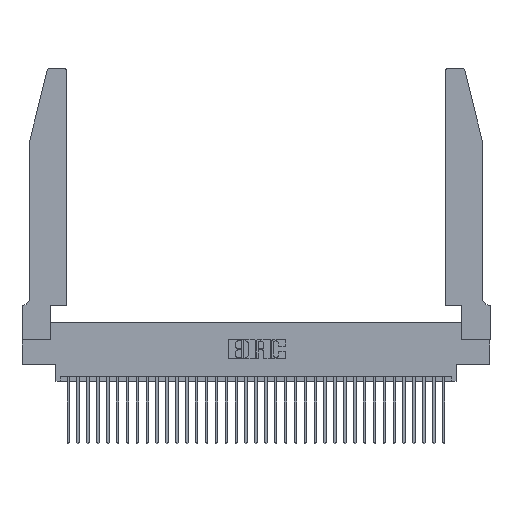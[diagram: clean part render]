
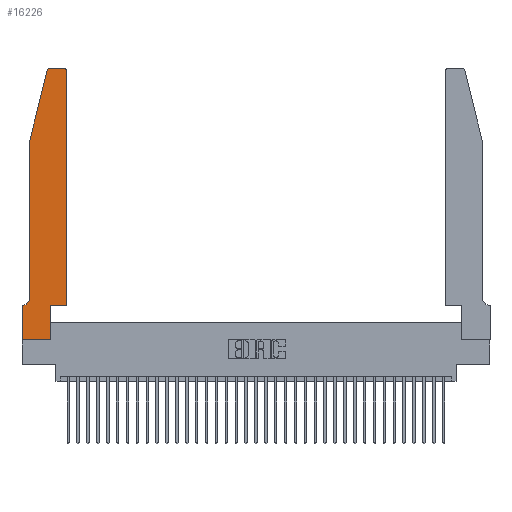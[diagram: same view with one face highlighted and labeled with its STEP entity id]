
A CAD part, top view. The second image highlights one B-rep face of the part: STEP entity #16226.
In plain terms, the highlighted planar face has unit normal (0, 0, 1).
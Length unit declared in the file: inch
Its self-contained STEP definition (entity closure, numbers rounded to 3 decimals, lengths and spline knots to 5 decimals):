
#442 = VERTEX_POINT ( 'NONE', #21804 ) ;
#1699 = ORIENTED_EDGE ( 'NONE', *, *, #30602, .T. ) ;
#1882 = AXIS2_PLACEMENT_3D ( 'NONE', #15471, #9802, #29701 ) ;
#3383 = EDGE_CURVE ( 'NONE', #442, #19058, #23968, .T. ) ;
#3510 = ORIENTED_EDGE ( 'NONE', *, *, #5748, .T. ) ;
#3733 = CARTESIAN_POINT ( 'NONE',  ( 0.4505, 0.35, 0.37 ) ) ;
#4186 = ORIENTED_EDGE ( 'NONE', *, *, #34453, .T. ) ;
#4573 = EDGE_CURVE ( 'NONE', #18616, #24923, #19539, .T. ) ;
#4771 = DIRECTION ( 'NONE',  ( -1., 0., 0. ) ) ;
#4941 = ORIENTED_EDGE ( 'NONE', *, *, #29154, .T. ) ;
#5039 = CARTESIAN_POINT ( 'NONE',  ( 0.0755, 0.42, 0.37 ) ) ;
#5607 = LINE ( 'NONE', #7741, #11614 ) ;
#5748 = EDGE_CURVE ( 'NONE', #34506, #9869, #10215, .T. ) ;
#7741 = CARTESIAN_POINT ( 'NONE',  ( 0., 0., 0.37 ) ) ;
#7830 = CARTESIAN_POINT ( 'NONE',  ( 0.2865, 0.35, 0.37 ) ) ;
#8473 = ORIENTED_EDGE ( 'NONE', *, *, #3383, .T. ) ;
#8929 = CIRCLE ( 'NONE', #1882, 0.03 ) ;
#9201 = AXIS2_PLACEMENT_3D ( 'NONE', #35450, #16114, #35322 ) ;
#9614 = ORIENTED_EDGE ( 'NONE', *, *, #13387, .T. ) ;
#9802 = DIRECTION ( 'NONE',  ( 0., 0., 1. ) ) ;
#9806 = EDGE_CURVE ( 'NONE', #19344, #442, #5607, .T. ) ;
#9869 = VERTEX_POINT ( 'NONE', #19408 ) ;
#10199 = DIRECTION ( 'NONE',  ( 0., 1., 0. ) ) ;
#10215 = CIRCLE ( 'NONE', #30961, 0.07 ) ;
#10326 = LINE ( 'NONE', #27011, #16774 ) ;
#10387 = DIRECTION ( 'NONE',  ( 1., 0., 0. ) ) ;
#10603 = ORIENTED_EDGE ( 'NONE', *, *, #4573, .T. ) ;
#10784 = CARTESIAN_POINT ( 'NONE',  ( 0.0755, 0.35, 0.37 ) ) ;
#11123 = CARTESIAN_POINT ( 'NONE',  ( 0.2865, 0., 0.37 ) ) ;
#11614 = VECTOR ( 'NONE', #23909, 39.37008 ) ;
#11925 = LINE ( 'NONE', #7830, #24583 ) ;
#12015 = CARTESIAN_POINT ( 'NONE',  ( 0.4505, 2.72, 0.37 ) ) ;
#12252 = DIRECTION ( 'NONE',  ( 1., 0., 0. ) ) ;
#12327 = EDGE_CURVE ( 'NONE', #34112, #19945, #30790, .T. ) ;
#12474 = LINE ( 'NONE', #20867, #32475 ) ;
#13083 = VERTEX_POINT ( 'NONE', #3733 ) ;
#13387 = EDGE_CURVE ( 'NONE', #13083, #19065, #12474, .T. ) ;
#14376 = ORIENTED_EDGE ( 'NONE', *, *, #12327, .T. ) ;
#14694 = CARTESIAN_POINT ( 'NONE',  ( 0., 0.35, 0.37 ) ) ;
#14725 = VECTOR ( 'NONE', #27027, 39.37008 ) ;
#14819 = CARTESIAN_POINT ( 'NONE',  ( 0.0755, 2., 0.37 ) ) ;
#14823 = LINE ( 'NONE', #19082, #28723 ) ;
#15471 = CARTESIAN_POINT ( 'NONE',  ( 0.284, 2.72, 0.37 ) ) ;
#16031 = VECTOR ( 'NONE', #4771, 39.37008 ) ;
#16114 = DIRECTION ( 'NONE',  ( 0., 0., 1. ) ) ;
#16217 = FACE_OUTER_BOUND ( 'NONE', #30870, .T. ) ;
#16226 = ADVANCED_FACE ( 'NONE', ( #16217 ), #17483, .T. ) ;
#16430 = DIRECTION ( 'NONE',  ( -1., 0., 0. ) ) ;
#16774 = VECTOR ( 'NONE', #32219, 39.37008 ) ;
#17483 = PLANE ( 'NONE',  #19609 ) ;
#18475 = CARTESIAN_POINT ( 'NONE',  ( 0.2865, 0.35, 0.37 ) ) ;
#18616 = VERTEX_POINT ( 'NONE', #30779 ) ;
#18651 = CARTESIAN_POINT ( 'NONE',  ( 0.0755, 2., 0.37 ) ) ;
#19058 = VERTEX_POINT ( 'NONE', #11123 ) ;
#19065 = VERTEX_POINT ( 'NONE', #12015 ) ;
#19082 = CARTESIAN_POINT ( 'NONE',  ( 0.4505, 0.35, 0.37 ) ) ;
#19344 = VERTEX_POINT ( 'NONE', #14694 ) ;
#19408 = CARTESIAN_POINT ( 'NONE',  ( 0.0055, 0.35, 0.37 ) ) ;
#19539 = LINE ( 'NONE', #18651, #14725 ) ;
#19571 = CARTESIAN_POINT ( 'NONE',  ( 0.4205, 2.75, 0.37 ) ) ;
#19609 = AXIS2_PLACEMENT_3D ( 'NONE', #20054, #34510, #29400 ) ;
#19945 = VERTEX_POINT ( 'NONE', #22219 ) ;
#20054 = CARTESIAN_POINT ( 'NONE',  ( 0., 0.35, 0.37 ) ) ;
#20576 = CARTESIAN_POINT ( 'NONE',  ( 0., 0., 0.37 ) ) ;
#20867 = CARTESIAN_POINT ( 'NONE',  ( 0.4505, 0.35, 0.37 ) ) ;
#21250 = DIRECTION ( 'NONE',  ( 0., 0., -1. ) ) ;
#21804 = CARTESIAN_POINT ( 'NONE',  ( 0., 0., 0.37 ) ) ;
#22219 = CARTESIAN_POINT ( 'NONE',  ( 0.284, 2.75, 0.37 ) ) ;
#22234 = EDGE_CURVE ( 'NONE', #24923, #34506, #10326, .T. ) ;
#22964 = ORIENTED_EDGE ( 'NONE', *, *, #22234, .T. ) ;
#23137 = LINE ( 'NONE', #10784, #35368 ) ;
#23337 = EDGE_CURVE ( 'NONE', #19945, #18616, #8929, .T. ) ;
#23909 = DIRECTION ( 'NONE',  ( 0., -1., 0. ) ) ;
#23968 = LINE ( 'NONE', #20576, #34844 ) ;
#23972 = EDGE_CURVE ( 'NONE', #9869, #19344, #23137, .T. ) ;
#24059 = CARTESIAN_POINT ( 'NONE',  ( 0.0055, 0.42, 0.37 ) ) ;
#24583 = VECTOR ( 'NONE', #10199, 39.37008 ) ;
#24923 = VERTEX_POINT ( 'NONE', #14819 ) ;
#26205 = DIRECTION ( 'NONE',  ( 0., 1., 0. ) ) ;
#26486 = ORIENTED_EDGE ( 'NONE', *, *, #23337, .T. ) ;
#27011 = CARTESIAN_POINT ( 'NONE',  ( 0.0755, 2., 0.37 ) ) ;
#27027 = DIRECTION ( 'NONE',  ( -0.239, -0.971, 0. ) ) ;
#28723 = VECTOR ( 'NONE', #10387, 39.37008 ) ;
#29050 = ORIENTED_EDGE ( 'NONE', *, *, #23972, .T. ) ;
#29154 = EDGE_CURVE ( 'NONE', #19058, #30435, #11925, .T. ) ;
#29400 = DIRECTION ( 'NONE',  ( 1., 0., 0. ) ) ;
#29701 = DIRECTION ( 'NONE',  ( 1., 0., 0. ) ) ;
#30435 = VERTEX_POINT ( 'NONE', #18475 ) ;
#30602 = EDGE_CURVE ( 'NONE', #30435, #13083, #14823, .T. ) ;
#30779 = CARTESIAN_POINT ( 'NONE',  ( 0.25487, 2.72718, 0.37 ) ) ;
#30790 = LINE ( 'NONE', #32501, #16031 ) ;
#30810 = CIRCLE ( 'NONE', #9201, 0.03 ) ;
#30870 = EDGE_LOOP ( 'NONE', ( #14376, #26486, #10603, #22964, #3510, #29050, #33937, #8473, #4941, #1699, #9614, #4186 ) ) ;
#30961 = AXIS2_PLACEMENT_3D ( 'NONE', #24059, #21250, #35644 ) ;
#32219 = DIRECTION ( 'NONE',  ( 0., -1., 0. ) ) ;
#32475 = VECTOR ( 'NONE', #26205, 39.37008 ) ;
#32501 = CARTESIAN_POINT ( 'NONE',  ( 0.2605, 2.75, 0.37 ) ) ;
#33937 = ORIENTED_EDGE ( 'NONE', *, *, #9806, .T. ) ;
#34112 = VERTEX_POINT ( 'NONE', #19571 ) ;
#34453 = EDGE_CURVE ( 'NONE', #19065, #34112, #30810, .T. ) ;
#34506 = VERTEX_POINT ( 'NONE', #5039 ) ;
#34510 = DIRECTION ( 'NONE',  ( 0., 0., 1. ) ) ;
#34844 = VECTOR ( 'NONE', #12252, 39.37008 ) ;
#35322 = DIRECTION ( 'NONE',  ( 1., 0., 0. ) ) ;
#35368 = VECTOR ( 'NONE', #16430, 39.37008 ) ;
#35450 = CARTESIAN_POINT ( 'NONE',  ( 0.4205, 2.72, 0.37 ) ) ;
#35644 = DIRECTION ( 'NONE',  ( -1., 0., 0. ) ) ;
